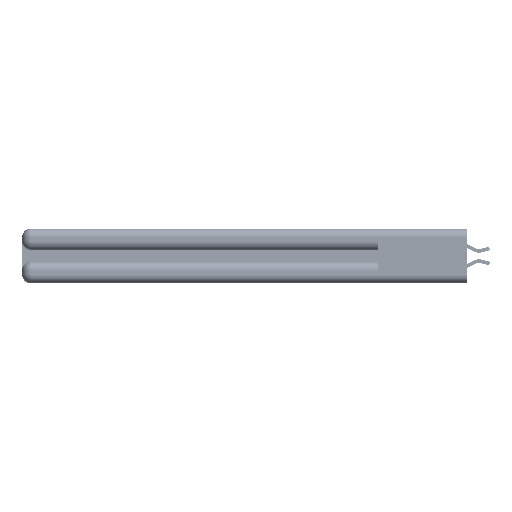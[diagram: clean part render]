
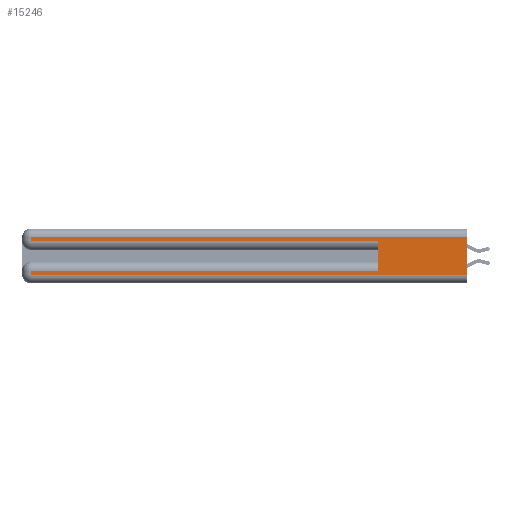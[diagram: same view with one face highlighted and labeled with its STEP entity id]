
A CAD part, left-side view. The second image highlights one B-rep face of the part: STEP entity #15246.
In plain terms, the highlighted planar face has unit normal (-1, 0, 0).
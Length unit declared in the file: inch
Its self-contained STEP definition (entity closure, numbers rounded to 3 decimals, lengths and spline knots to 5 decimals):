
#516 = CARTESIAN_POINT ( 'NONE',  ( 0., 0.6, 0.285 ) ) ;
#2575 = DIRECTION ( 'NONE',  ( 0., 0., -1. ) ) ;
#2847 = EDGE_CURVE ( 'NONE', #22632, #15027, #11382, .T. ) ;
#4764 = DIRECTION ( 'NONE',  ( 0., 0., -1. ) ) ;
#6370 = DIRECTION ( 'NONE',  ( 1., 0., 0. ) ) ;
#6861 = PLANE ( 'NONE',  #47697 ) ;
#7467 = DIRECTION ( 'NONE',  ( 0., 1., 0. ) ) ;
#8315 = CARTESIAN_POINT ( 'NONE',  ( 0., 2.94, 0.37 ) ) ;
#8421 = ORIENTED_EDGE ( 'NONE', *, *, #22629, .T. ) ;
#8542 = EDGE_LOOP ( 'NONE', ( #43636, #8421, #20145, #34942, #13839, #48440, #29021, #33496 ) ) ;
#9226 = VERTEX_POINT ( 'NONE', #43944 ) ;
#9821 = VECTOR ( 'NONE', #36753, 39.37008 ) ;
#11012 = VERTEX_POINT ( 'NONE', #29113 ) ;
#11382 = LINE ( 'NONE', #35085, #14429 ) ;
#12100 = LINE ( 'NONE', #15509, #31713 ) ;
#13074 = EDGE_CURVE ( 'NONE', #22632, #9226, #16211, .T. ) ;
#13656 = VERTEX_POINT ( 'NONE', #29749 ) ;
#13839 = ORIENTED_EDGE ( 'NONE', *, *, #2847, .F. ) ;
#14004 = LINE ( 'NONE', #28196, #39732 ) ;
#14429 = VECTOR ( 'NONE', #50690, 39.37008 ) ;
#15027 = VERTEX_POINT ( 'NONE', #516 ) ;
#15246 = ADVANCED_FACE ( 'NONE', ( #24156 ), #6861, .F. ) ;
#15509 = CARTESIAN_POINT ( 'NONE',  ( 0., 0., 0.31 ) ) ;
#16211 = LINE ( 'NONE', #22292, #50497 ) ;
#16439 = LINE ( 'NONE', #8315, #42183 ) ;
#16552 = CARTESIAN_POINT ( 'NONE',  ( 0., 0., 0.06 ) ) ;
#18153 = CARTESIAN_POINT ( 'NONE',  ( 0., 2.94, 0.285 ) ) ;
#18526 = VECTOR ( 'NONE', #45490, 39.37008 ) ;
#19465 = CARTESIAN_POINT ( 'NONE',  ( 0., 0.6, 0.085 ) ) ;
#20145 = ORIENTED_EDGE ( 'NONE', *, *, #22084, .T. ) ;
#21240 = LINE ( 'NONE', #16552, #47522 ) ;
#22084 = EDGE_CURVE ( 'NONE', #11012, #46514, #14004, .T. ) ;
#22292 = CARTESIAN_POINT ( 'NONE',  ( 0., 0., 0.085 ) ) ;
#22629 = EDGE_CURVE ( 'NONE', #13656, #11012, #12100, .T. ) ;
#22632 = VERTEX_POINT ( 'NONE', #19465 ) ;
#23740 = CARTESIAN_POINT ( 'NONE',  ( 0., 0., 0.06 ) ) ;
#24156 = FACE_OUTER_BOUND ( 'NONE', #8542, .T. ) ;
#25495 = CARTESIAN_POINT ( 'NONE',  ( 0., 0., 0.37 ) ) ;
#27635 = DIRECTION ( 'NONE',  ( 0., 0., -1. ) ) ;
#28196 = CARTESIAN_POINT ( 'NONE',  ( 0., 2.94, 0.37 ) ) ;
#28868 = DIRECTION ( 'NONE',  ( 0., -1., 0. ) ) ;
#29021 = ORIENTED_EDGE ( 'NONE', *, *, #45717, .T. ) ;
#29113 = CARTESIAN_POINT ( 'NONE',  ( 0., 2.94, 0.31 ) ) ;
#29749 = CARTESIAN_POINT ( 'NONE',  ( 0., 0., 0.31 ) ) ;
#31713 = VECTOR ( 'NONE', #7467, 39.37008 ) ;
#33496 = ORIENTED_EDGE ( 'NONE', *, *, #38787, .T. ) ;
#33835 = LINE ( 'NONE', #25495, #18526 ) ;
#34942 = ORIENTED_EDGE ( 'NONE', *, *, #50491, .T. ) ;
#35085 = CARTESIAN_POINT ( 'NONE',  ( 0., 0.6, 0.145 ) ) ;
#35320 = EDGE_CURVE ( 'NONE', #13656, #45685, #33835, .T. ) ;
#36753 = DIRECTION ( 'NONE',  ( 0., -1., 0. ) ) ;
#37308 = LINE ( 'NONE', #41223, #9821 ) ;
#38155 = CARTESIAN_POINT ( 'NONE',  ( 0., 0., 0.37 ) ) ;
#38787 = EDGE_CURVE ( 'NONE', #41317, #45685, #21240, .T. ) ;
#39732 = VECTOR ( 'NONE', #4764, 39.37008 ) ;
#41223 = CARTESIAN_POINT ( 'NONE',  ( 0., 0., 0.285 ) ) ;
#41317 = VERTEX_POINT ( 'NONE', #43050 ) ;
#41955 = DIRECTION ( 'NONE',  ( 0., 1., 0. ) ) ;
#42183 = VECTOR ( 'NONE', #27635, 39.37008 ) ;
#43050 = CARTESIAN_POINT ( 'NONE',  ( 0., 2.94, 0.06 ) ) ;
#43636 = ORIENTED_EDGE ( 'NONE', *, *, #35320, .F. ) ;
#43944 = CARTESIAN_POINT ( 'NONE',  ( 0., 2.94, 0.085 ) ) ;
#45490 = DIRECTION ( 'NONE',  ( 0., 0., -1. ) ) ;
#45685 = VERTEX_POINT ( 'NONE', #23740 ) ;
#45717 = EDGE_CURVE ( 'NONE', #9226, #41317, #16439, .T. ) ;
#46514 = VERTEX_POINT ( 'NONE', #18153 ) ;
#47522 = VECTOR ( 'NONE', #28868, 39.37008 ) ;
#47697 = AXIS2_PLACEMENT_3D ( 'NONE', #38155, #6370, #2575 ) ;
#48440 = ORIENTED_EDGE ( 'NONE', *, *, #13074, .T. ) ;
#50491 = EDGE_CURVE ( 'NONE', #46514, #15027, #37308, .T. ) ;
#50497 = VECTOR ( 'NONE', #41955, 39.37008 ) ;
#50690 = DIRECTION ( 'NONE',  ( 0., 0., 1. ) ) ;
